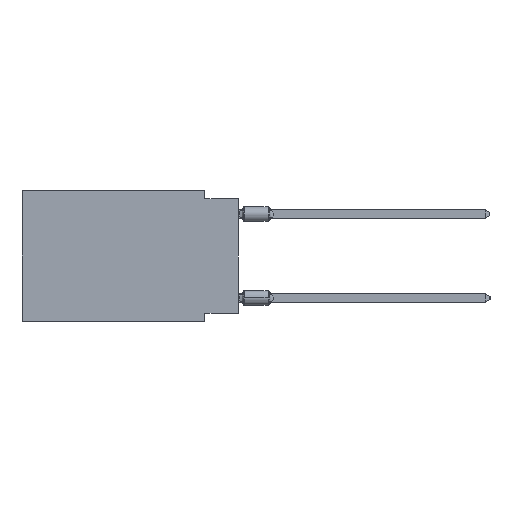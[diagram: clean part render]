
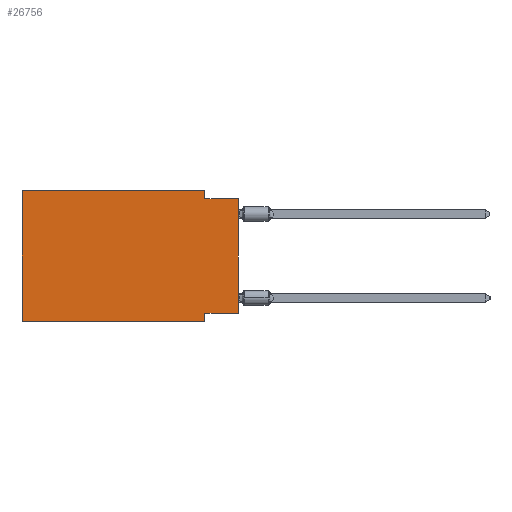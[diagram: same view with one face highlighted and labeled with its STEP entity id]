
A CAD part, left-side view. The second image highlights one B-rep face of the part: STEP entity #26756.
In plain terms, the highlighted planar face has unit normal (-1, 0, 0).
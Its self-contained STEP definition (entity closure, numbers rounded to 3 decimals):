
#600 = LINE ( 'NONE', #18583, #35857 ) ;
#1599 = ORIENTED_EDGE ( 'NONE', *, *, #3397, .T. ) ;
#2297 = CARTESIAN_POINT ( 'NONE',  ( 0., 16.383, 0. ) ) ;
#3397 = EDGE_CURVE ( 'NONE', #45766, #40062, #600, .T. ) ;
#3992 = DIRECTION ( 'NONE',  ( 1., 0., 0. ) ) ;
#6577 = EDGE_CURVE ( 'NONE', #17471, #37865, #15328, .T. ) ;
#7984 = VECTOR ( 'NONE', #29256, 1000. ) ;
#8561 = PLANE ( 'NONE',  #19080 ) ;
#8743 = CARTESIAN_POINT ( 'NONE',  ( 0., 16.383, 0. ) ) ;
#9921 = DIRECTION ( 'NONE',  ( 0., 1., 0. ) ) ;
#11022 = EDGE_CURVE ( 'NONE', #37865, #40062, #52445, .T. ) ;
#11271 = CARTESIAN_POINT ( 'NONE',  ( 0., 16.383, -9.906 ) ) ;
#11852 = CARTESIAN_POINT ( 'NONE',  ( 0., 0., 0. ) ) ;
#15165 = CARTESIAN_POINT ( 'NONE',  ( 0., 2.54, 0. ) ) ;
#15328 = LINE ( 'NONE', #32741, #19552 ) ;
#16353 = DIRECTION ( 'NONE',  ( 0., 0., 1. ) ) ;
#17053 = CARTESIAN_POINT ( 'NONE',  ( 0., 2.54, 0. ) ) ;
#17471 = VERTEX_POINT ( 'NONE', #46042 ) ;
#18480 = CARTESIAN_POINT ( 'NONE',  ( 0., 2.54, -9.906 ) ) ;
#18583 = CARTESIAN_POINT ( 'NONE',  ( 0., 16.383, -9.906 ) ) ;
#19080 = AXIS2_PLACEMENT_3D ( 'NONE', #43101, #3992, #38818 ) ;
#19309 = CARTESIAN_POINT ( 'NONE',  ( 0., 16.383, 0. ) ) ;
#19552 = VECTOR ( 'NONE', #9921, 1000. ) ;
#19680 = CARTESIAN_POINT ( 'NONE',  ( 0., 2.54, -0.635 ) ) ;
#20560 = ORIENTED_EDGE ( 'NONE', *, *, #37566, .F. ) ;
#21034 = VECTOR ( 'NONE', #43633, 1000. ) ;
#23071 = EDGE_CURVE ( 'NONE', #17471, #30343, #34105, .T. ) ;
#23735 = VERTEX_POINT ( 'NONE', #15165 ) ;
#24774 = LINE ( 'NONE', #17053, #45476 ) ;
#25151 = EDGE_LOOP ( 'NONE', ( #53176, #45559, #51627, #20560, #48057, #1599, #45793, #50779 ) ) ;
#26098 = EDGE_CURVE ( 'NONE', #45766, #41209, #55161, .T. ) ;
#26155 = DIRECTION ( 'NONE',  ( 0., -1., 0. ) ) ;
#26756 = ADVANCED_FACE ( 'NONE', ( #29964 ), #8561, .F. ) ;
#29256 = DIRECTION ( 'NONE',  ( 0., 0., 1. ) ) ;
#29939 = CARTESIAN_POINT ( 'NONE',  ( 0., 0., -0.635 ) ) ;
#29964 = FACE_OUTER_BOUND ( 'NONE', #25151, .T. ) ;
#30055 = VECTOR ( 'NONE', #40750, 1000. ) ;
#30329 = VECTOR ( 'NONE', #26155, 1000. ) ;
#30343 = VERTEX_POINT ( 'NONE', #39513 ) ;
#30655 = CARTESIAN_POINT ( 'NONE',  ( 0., 2.54, -9.271 ) ) ;
#32234 = CARTESIAN_POINT ( 'NONE',  ( 0., 2.54, -9.906 ) ) ;
#32728 = EDGE_CURVE ( 'NONE', #23735, #52110, #24774, .T. ) ;
#32741 = CARTESIAN_POINT ( 'NONE',  ( 0., 0., -9.271 ) ) ;
#34105 = LINE ( 'NONE', #11852, #7984 ) ;
#35857 = VECTOR ( 'NONE', #43415, 1000. ) ;
#37566 = EDGE_CURVE ( 'NONE', #41209, #23735, #52125, .T. ) ;
#37865 = VERTEX_POINT ( 'NONE', #30655 ) ;
#38305 = VECTOR ( 'NONE', #16353, 1000. ) ;
#38466 = DIRECTION ( 'NONE',  ( 0., 0., -1. ) ) ;
#38818 = DIRECTION ( 'NONE',  ( 0., 0., -1. ) ) ;
#39513 = CARTESIAN_POINT ( 'NONE',  ( 0., 0., -0.635 ) ) ;
#40062 = VERTEX_POINT ( 'NONE', #32234 ) ;
#40750 = DIRECTION ( 'NONE',  ( 0., 0., -1. ) ) ;
#41209 = VERTEX_POINT ( 'NONE', #2297 ) ;
#41497 = EDGE_CURVE ( 'NONE', #52110, #30343, #43354, .T. ) ;
#43101 = CARTESIAN_POINT ( 'NONE',  ( 0., 16.383, 0. ) ) ;
#43354 = LINE ( 'NONE', #29939, #21034 ) ;
#43415 = DIRECTION ( 'NONE',  ( 0., -1., 0. ) ) ;
#43633 = DIRECTION ( 'NONE',  ( 0., -1., 0. ) ) ;
#45476 = VECTOR ( 'NONE', #38466, 1000. ) ;
#45559 = ORIENTED_EDGE ( 'NONE', *, *, #41497, .F. ) ;
#45766 = VERTEX_POINT ( 'NONE', #11271 ) ;
#45793 = ORIENTED_EDGE ( 'NONE', *, *, #11022, .F. ) ;
#46042 = CARTESIAN_POINT ( 'NONE',  ( 0., 0., -9.271 ) ) ;
#48057 = ORIENTED_EDGE ( 'NONE', *, *, #26098, .F. ) ;
#50779 = ORIENTED_EDGE ( 'NONE', *, *, #6577, .F. ) ;
#51627 = ORIENTED_EDGE ( 'NONE', *, *, #32728, .F. ) ;
#52110 = VERTEX_POINT ( 'NONE', #19680 ) ;
#52125 = LINE ( 'NONE', #8743, #30329 ) ;
#52445 = LINE ( 'NONE', #18480, #30055 ) ;
#53176 = ORIENTED_EDGE ( 'NONE', *, *, #23071, .T. ) ;
#55161 = LINE ( 'NONE', #19309, #38305 ) ;
